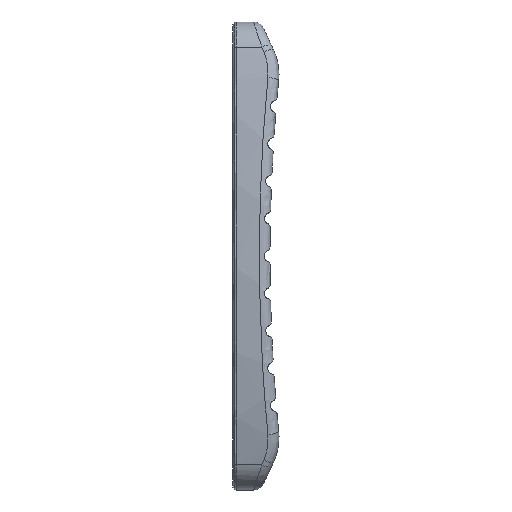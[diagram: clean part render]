
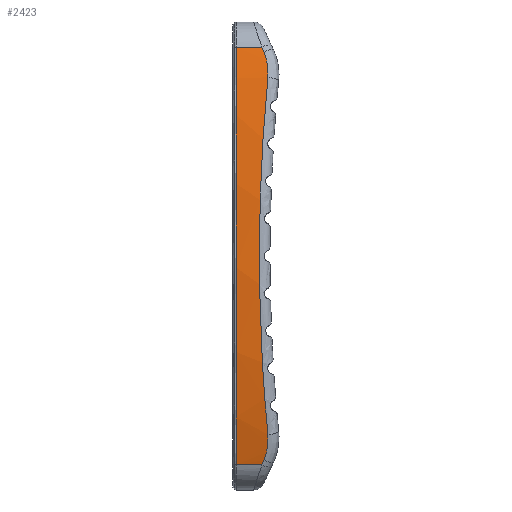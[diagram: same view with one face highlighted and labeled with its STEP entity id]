
A CAD part, left-side view. The second image highlights one B-rep face of the part: STEP entity #2423.
In plain terms, the highlighted free-form (B-spline) face has degree [1, 2] with [2, 5] control points.
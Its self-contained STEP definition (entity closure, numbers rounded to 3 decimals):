
#47=(
BOUNDED_SURFACE()
B_SPLINE_SURFACE(1,2,((#7209,#7210,#7211,#7212,#7213),(#7214,#7215,#7216,
#7217,#7218)),.UNSPECIFIED.,.F.,.F.,.F.)
B_SPLINE_SURFACE_WITH_KNOTS((2,2),(3,2,3),(-0.018,0.103),
(-2.476,-1.571,-0.665),.UNSPECIFIED.)
GEOMETRIC_REPRESENTATION_ITEM()
RATIONAL_B_SPLINE_SURFACE(((1.,0.899,1.,0.899,1.),
(1.,0.899,1.,0.899,1.)))
REPRESENTATION_ITEM('')
SURFACE()
);
#162=LINE('',#6140,#258);
#184=LINE('',#7208,#280);
#258=VECTOR('',#2942,10.);
#280=VECTOR('',#3026,10.);
#421=FACE_OUTER_BOUND('',#581,.T.);
#581=EDGE_LOOP('',(#2042,#2043,#2044,#2045,#2046,#2047,#2048,#2049));
#744=B_SPLINE_CURVE_WITH_KNOTS('',3,(#6195,#6196,#6197,#6198),
 .UNSPECIFIED.,.F.,.F.,(4,4),(-0.128,0.),.UNSPECIFIED.);
#747=B_SPLINE_CURVE_WITH_KNOTS('',3,(#6231,#6232,#6233,#6234),
 .UNSPECIFIED.,.F.,.F.,(4,4),(0.,0.668),.UNSPECIFIED.);
#751=B_SPLINE_CURVE_WITH_KNOTS('',3,(#6310,#6311,#6312,#6313),
 .UNSPECIFIED.,.F.,.F.,(4,4),(-0.128,0.),.UNSPECIFIED.);
#753=B_SPLINE_CURVE_WITH_KNOTS('',3,(#6340,#6341,#6342,#6343),
 .UNSPECIFIED.,.F.,.F.,(4,4),(0.,0.668),.UNSPECIFIED.);
#790=B_SPLINE_CURVE_WITH_KNOTS('',3,(#7133,#7134,#7135,#7136,#7137,#7138,
#7139,#7140),.UNSPECIFIED.,.F.,.F.,(4,1,1,1,1,4),(-10.219,-8.932,
-7.645,-5.071,-2.497,-1.21),
 .UNSPECIFIED.);
#792=B_SPLINE_CURVE_WITH_KNOTS('',3,(#7219,#7220,#7221,#7222,#7223,#7224,
#7225,#7226,#7227,#7228,#7229),.UNSPECIFIED.,.F.,.F.,(4,1,1,1,1,1,1,1,4),
(0.,0.763,1.525,3.05,4.575,
7.626,9.151,9.913,10.676),
 .UNSPECIFIED.);
#1057=VERTEX_POINT('',#6136);
#1059=VERTEX_POINT('',#6139);
#1063=VERTEX_POINT('',#6194);
#1065=VERTEX_POINT('',#6225);
#1071=VERTEX_POINT('',#6280);
#1073=VERTEX_POINT('',#6308);
#1074=VERTEX_POINT('',#6334);
#1114=VERTEX_POINT('',#7206);
#1361=EDGE_CURVE('',#1057,#1059,#162,.T.);
#1367=EDGE_CURVE('',#1059,#1063,#744,.T.);
#1372=EDGE_CURVE('',#1063,#1065,#747,.T.);
#1384=EDGE_CURVE('',#1071,#1073,#751,.T.);
#1386=EDGE_CURVE('',#1073,#1074,#753,.T.);
#1432=EDGE_CURVE('',#1065,#1074,#790,.T.);
#1445=EDGE_CURVE('',#1114,#1071,#184,.T.);
#1446=EDGE_CURVE('',#1114,#1057,#792,.T.);
#2042=ORIENTED_EDGE('',*,*,#1446,.F.);
#2043=ORIENTED_EDGE('',*,*,#1445,.T.);
#2044=ORIENTED_EDGE('',*,*,#1384,.T.);
#2045=ORIENTED_EDGE('',*,*,#1386,.T.);
#2046=ORIENTED_EDGE('',*,*,#1432,.F.);
#2047=ORIENTED_EDGE('',*,*,#1372,.F.);
#2048=ORIENTED_EDGE('',*,*,#1367,.F.);
#2049=ORIENTED_EDGE('',*,*,#1361,.F.);
#2423=ADVANCED_FACE('',(#421),#47,.F.);
#2942=DIRECTION('',(0.,-1.,0.));
#3026=DIRECTION('',(0.,-1.,0.));
#6136=CARTESIAN_POINT('',(-10.031,-696.266,133.253));
#6139=CARTESIAN_POINT('',(-10.031,-702.77,133.253));
#6140=CARTESIAN_POINT('',(-10.031,-697.501,133.253));
#6194=CARTESIAN_POINT('',(-10.379,-703.287,132.088));
#6195=CARTESIAN_POINT('Ctrl Pts',(-10.031,-702.77,133.253));
#6196=CARTESIAN_POINT('Ctrl Pts',(-10.15,-702.942,132.865));
#6197=CARTESIAN_POINT('Ctrl Pts',(-10.266,-703.114,132.477));
#6198=CARTESIAN_POINT('Ctrl Pts',(-10.379,-703.287,132.088));
#6225=CARTESIAN_POINT('',(-12.022,-704.35,125.587));
#6231=CARTESIAN_POINT('Ctrl Pts',(-10.379,-703.287,132.088));
#6232=CARTESIAN_POINT('Ctrl Pts',(-10.968,-704.188,130.064));
#6233=CARTESIAN_POINT('Ctrl Pts',(-11.535,-704.564,127.803));
#6234=CARTESIAN_POINT('Ctrl Pts',(-12.022,-704.35,125.587));
#6280=CARTESIAN_POINT('',(-10.031,-702.77,27.353));
#6308=CARTESIAN_POINT('',(-10.379,-703.287,28.518));
#6310=CARTESIAN_POINT('Ctrl Pts',(-10.031,-702.77,27.353));
#6311=CARTESIAN_POINT('Ctrl Pts',(-10.15,-702.942,27.741));
#6312=CARTESIAN_POINT('Ctrl Pts',(-10.266,-703.114,28.13));
#6313=CARTESIAN_POINT('Ctrl Pts',(-10.379,-703.287,28.518));
#6334=CARTESIAN_POINT('',(-12.022,-704.35,35.019));
#6340=CARTESIAN_POINT('Ctrl Pts',(-10.379,-703.287,28.518));
#6341=CARTESIAN_POINT('Ctrl Pts',(-10.968,-704.188,30.542));
#6342=CARTESIAN_POINT('Ctrl Pts',(-11.535,-704.564,32.804));
#6343=CARTESIAN_POINT('Ctrl Pts',(-12.022,-704.35,35.019));
#7133=CARTESIAN_POINT('Ctrl Pts',(-12.022,-704.35,125.587));
#7134=CARTESIAN_POINT('Ctrl Pts',(-12.959,-703.94,121.319));
#7135=CARTESIAN_POINT('Ctrl Pts',(-14.384,-703.225,112.736));
#7136=CARTESIAN_POINT('Ctrl Pts',(-16.093,-702.262,95.473));
#7137=CARTESIAN_POINT('Ctrl Pts',(-16.561,-701.957,73.794));
#7138=CARTESIAN_POINT('Ctrl Pts',(-15.083,-702.868,52.15));
#7139=CARTESIAN_POINT('Ctrl Pts',(-12.958,-703.94,39.284));
#7140=CARTESIAN_POINT('Ctrl Pts',(-12.022,-704.35,35.019));
#7206=CARTESIAN_POINT('',(-10.031,-696.266,27.353));
#7208=CARTESIAN_POINT('',(-10.031,-697.501,27.353));
#7209=CARTESIAN_POINT('Ctrl Pts',(-10.031,-696.266,133.253));
#7210=CARTESIAN_POINT('Ctrl Pts',(-16.25,-696.266,113.043));
#7211=CARTESIAN_POINT('Ctrl Pts',(-16.25,-696.266,80.303));
#7212=CARTESIAN_POINT('Ctrl Pts',(-16.25,-696.266,47.563));
#7213=CARTESIAN_POINT('Ctrl Pts',(-10.031,-696.266,27.353));
#7214=CARTESIAN_POINT('Ctrl Pts',(-10.031,-704.456,133.253));
#7215=CARTESIAN_POINT('Ctrl Pts',(-16.25,-704.456,113.043));
#7216=CARTESIAN_POINT('Ctrl Pts',(-16.25,-704.456,80.303));
#7217=CARTESIAN_POINT('Ctrl Pts',(-16.25,-704.456,47.563));
#7218=CARTESIAN_POINT('Ctrl Pts',(-10.031,-704.456,27.353));
#7219=CARTESIAN_POINT('Ctrl Pts',(-10.031,-696.266,27.353));
#7220=CARTESIAN_POINT('Ctrl Pts',(-10.782,-696.266,29.795));
#7221=CARTESIAN_POINT('Ctrl Pts',(-12.045,-696.266,34.748));
#7222=CARTESIAN_POINT('Ctrl Pts',(-13.936,-696.266,44.763));
#7223=CARTESIAN_POINT('Ctrl Pts',(-15.446,-696.266,57.425));
#7224=CARTESIAN_POINT('Ctrl Pts',(-16.558,-696.266,77.752));
#7225=CARTESIAN_POINT('Ctrl Pts',(-16.032,-696.266,98.148));
#7226=CARTESIAN_POINT('Ctrl Pts',(-13.94,-696.266,115.836));
#7227=CARTESIAN_POINT('Ctrl Pts',(-12.043,-696.266,125.862));
#7228=CARTESIAN_POINT('Ctrl Pts',(-10.782,-696.266,130.811));
#7229=CARTESIAN_POINT('Ctrl Pts',(-10.031,-696.266,133.253));
